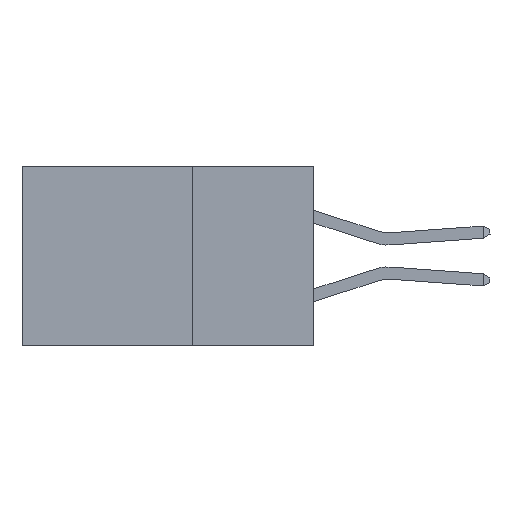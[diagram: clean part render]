
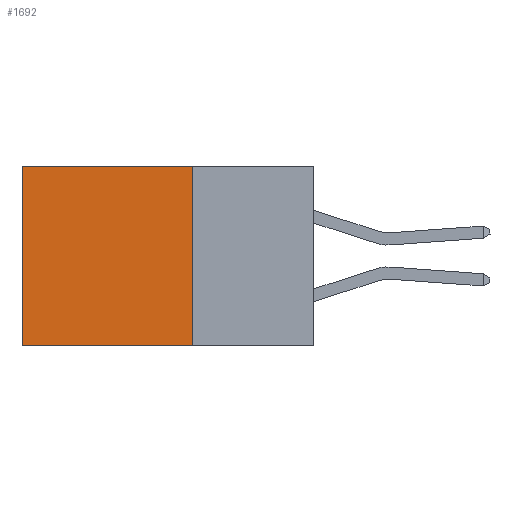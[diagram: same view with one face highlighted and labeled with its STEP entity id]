
A CAD part, left-side view. The second image highlights one B-rep face of the part: STEP entity #1692.
In plain terms, the highlighted planar face has unit normal (-1, 0, 0).
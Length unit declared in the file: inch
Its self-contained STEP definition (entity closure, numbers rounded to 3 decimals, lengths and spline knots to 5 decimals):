
#745 = FACE_OUTER_BOUND ( 'NONE', #831, .T. ) ;
#823 = VERTEX_POINT ( 'NONE', #4610 ) ;
#831 = EDGE_LOOP ( 'NONE', ( #11032, #6130, #7656, #3218 ) ) ;
#1173 = CARTESIAN_POINT ( 'NONE',  ( 0.2875, 0.6, -0.37 ) ) ;
#1286 = CARTESIAN_POINT ( 'NONE',  ( 0.2875, 0.25, 0. ) ) ;
#1320 = VECTOR ( 'NONE', #1372, 39.37008 ) ;
#1372 = DIRECTION ( 'NONE',  ( 0., 0., -1. ) ) ;
#1556 = CARTESIAN_POINT ( 'NONE',  ( 0.2875, 0.25, 0. ) ) ;
#1692 = ADVANCED_FACE ( 'NONE', ( #745 ), #2424, .F. ) ;
#2321 = LINE ( 'NONE', #1286, #1320 ) ;
#2424 = PLANE ( 'NONE',  #5767 ) ;
#2438 = LINE ( 'NONE', #8591, #11401 ) ;
#2466 = CARTESIAN_POINT ( 'NONE',  ( 0.2875, 0.25, 0. ) ) ;
#3218 = ORIENTED_EDGE ( 'NONE', *, *, #9583, .T. ) ;
#3788 = VERTEX_POINT ( 'NONE', #5451 ) ;
#3844 = VECTOR ( 'NONE', #8301, 39.37008 ) ;
#4584 = DIRECTION ( 'NONE',  ( 0., 1., 0. ) ) ;
#4610 = CARTESIAN_POINT ( 'NONE',  ( 0.2875, 0.6, 0. ) ) ;
#5451 = CARTESIAN_POINT ( 'NONE',  ( 0.2875, 0.25, -0.37 ) ) ;
#5767 = AXIS2_PLACEMENT_3D ( 'NONE', #1556, #8643, #9398 ) ;
#5989 = EDGE_CURVE ( 'NONE', #3788, #6265, #9064, .T. ) ;
#6130 = ORIENTED_EDGE ( 'NONE', *, *, #5989, .F. ) ;
#6265 = VERTEX_POINT ( 'NONE', #1173 ) ;
#6709 = DIRECTION ( 'NONE',  ( 0., 1., 0. ) ) ;
#7656 = ORIENTED_EDGE ( 'NONE', *, *, #8743, .F. ) ;
#7853 = LINE ( 'NONE', #10985, #3844 ) ;
#8098 = CARTESIAN_POINT ( 'NONE',  ( 0.2875, 0.25, -0.37 ) ) ;
#8219 = VERTEX_POINT ( 'NONE', #2466 ) ;
#8301 = DIRECTION ( 'NONE',  ( 0., 0., -1. ) ) ;
#8591 = CARTESIAN_POINT ( 'NONE',  ( 0.2875, 0.25, 0. ) ) ;
#8643 = DIRECTION ( 'NONE',  ( 1., 0., 0. ) ) ;
#8743 = EDGE_CURVE ( 'NONE', #8219, #3788, #2321, .T. ) ;
#9064 = LINE ( 'NONE', #8098, #10620 ) ;
#9398 = DIRECTION ( 'NONE',  ( 0., 0., -1. ) ) ;
#9583 = EDGE_CURVE ( 'NONE', #8219, #823, #2438, .T. ) ;
#9971 = EDGE_CURVE ( 'NONE', #823, #6265, #7853, .T. ) ;
#10620 = VECTOR ( 'NONE', #4584, 39.37008 ) ;
#10985 = CARTESIAN_POINT ( 'NONE',  ( 0.2875, 0.6, 0. ) ) ;
#11032 = ORIENTED_EDGE ( 'NONE', *, *, #9971, .T. ) ;
#11401 = VECTOR ( 'NONE', #6709, 39.37008 ) ;
